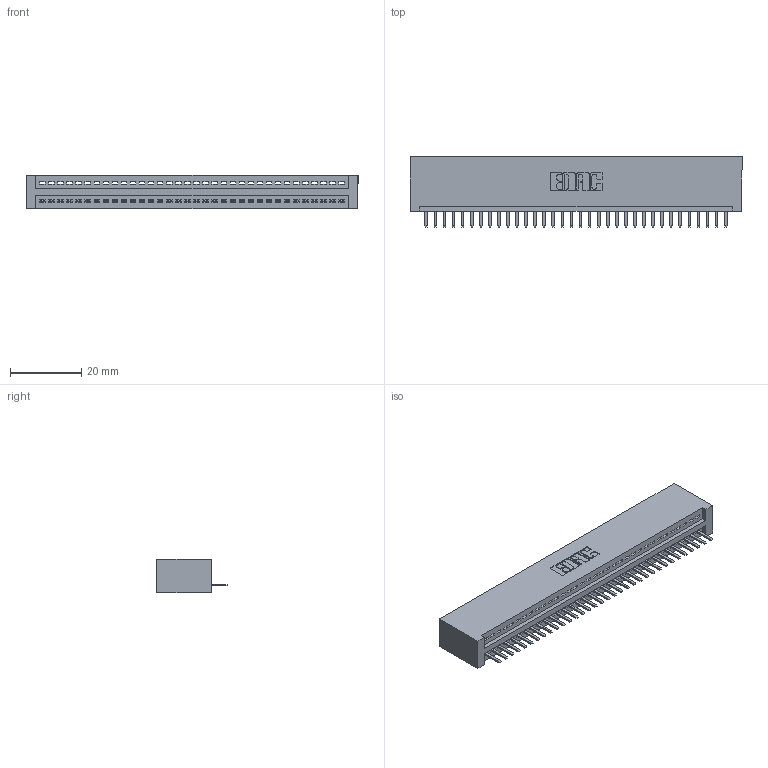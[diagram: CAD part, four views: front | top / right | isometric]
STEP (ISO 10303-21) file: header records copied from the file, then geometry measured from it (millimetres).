
FILE_DESCRIPTION (( 'STEP AP203' ), '1' );
FILE_NAME ('395-034-520-101.STEP', '2019-10-19T16:44:11', ( '' ), ( '' ), 'SwSTEP 2.0', 'SolidWorks 2016', '' );
FILE_SCHEMA (( 'CONFIG_CONTROL_DESIGN' ));
Length unit declared in the file: inch
Products named in the file (3): 345-292-001_345-293-120; 345 Part_No Mounting Lugs; 395-034-520-101
Assembly tree (35 placements, depth 2):
  395-034-520-101
    345 Part_No Mounting Lugs
    345-292-001_345-293-120  x34
Bounding box: 92.96 x 19.68 x 9.4 mm (x, y, z)
Volume: 9250.8 mm3; surface area: 12055 mm2
Topology: 35 solids, 35 shells, 2226 faces, 6573 edges, 4290 vertices
Faces by surface type: plane 1504, cylinder 722
Entity records: 26503 total; most frequent: CARTESIAN_POINT 4610, ORIENTED_EDGE 4566, DIRECTION 4019, EDGE_CURVE 2283, LINE 2019, VECTOR 2019, VERTEX_POINT 1518, AXIS2_PLACEMENT_3D 1000
